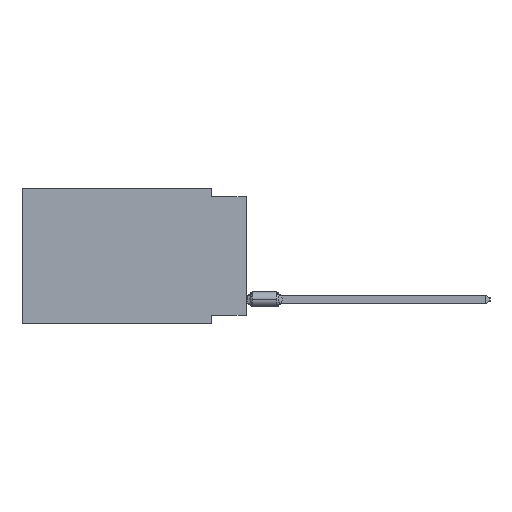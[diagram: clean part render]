
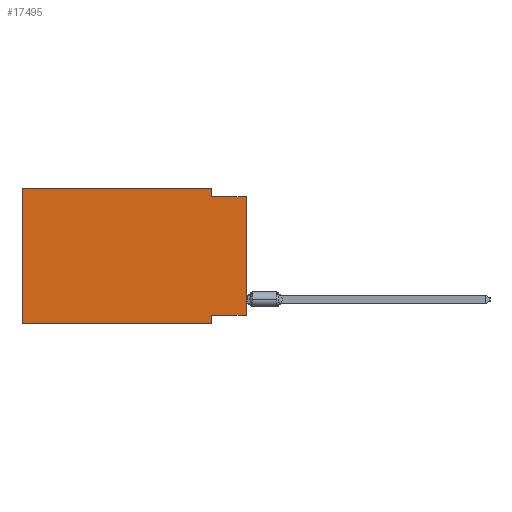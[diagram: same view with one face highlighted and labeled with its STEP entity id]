
A CAD part, left-side view. The second image highlights one B-rep face of the part: STEP entity #17495.
In plain terms, the highlighted planar face has unit normal (-1, 0, 0).
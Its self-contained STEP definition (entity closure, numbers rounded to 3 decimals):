
#126 = VERTEX_POINT ( 'NONE', #58675 ) ;
#635 = VERTEX_POINT ( 'NONE', #7079 ) ;
#2774 = CARTESIAN_POINT ( 'NONE',  ( 0., 0., -9.271 ) ) ;
#3363 = EDGE_CURVE ( 'NONE', #635, #11653, #28227, .T. ) ;
#3423 = LINE ( 'NONE', #3728, #13089 ) ;
#3728 = CARTESIAN_POINT ( 'NONE',  ( 0., 16.383, 0. ) ) ;
#4546 = ORIENTED_EDGE ( 'NONE', *, *, #44623, .F. ) ;
#6617 = AXIS2_PLACEMENT_3D ( 'NONE', #57399, #61791, #23849 ) ;
#7079 = CARTESIAN_POINT ( 'NONE',  ( 0., 2.54, -9.271 ) ) ;
#9538 = DIRECTION ( 'NONE',  ( 0., -1., 0. ) ) ;
#10046 = CARTESIAN_POINT ( 'NONE',  ( 0., 0., 0. ) ) ;
#10373 = DIRECTION ( 'NONE',  ( 0., 0., 1. ) ) ;
#10592 = CARTESIAN_POINT ( 'NONE',  ( 0., 2.54, 0. ) ) ;
#11311 = ORIENTED_EDGE ( 'NONE', *, *, #11532, .F. ) ;
#11532 = EDGE_CURVE ( 'NONE', #30861, #30033, #38598, .T. ) ;
#11653 = VERTEX_POINT ( 'NONE', #49554 ) ;
#12289 = VERTEX_POINT ( 'NONE', #34632 ) ;
#13089 = VECTOR ( 'NONE', #22614, 1000. ) ;
#13993 = LINE ( 'NONE', #18708, #18379 ) ;
#14988 = DIRECTION ( 'NONE',  ( 0., -1., 0. ) ) ;
#15938 = CARTESIAN_POINT ( 'NONE',  ( 0., 0., -0.635 ) ) ;
#17495 = ADVANCED_FACE ( 'NONE', ( #47383 ), #42677, .F. ) ;
#18379 = VECTOR ( 'NONE', #28171, 1000. ) ;
#18708 = CARTESIAN_POINT ( 'NONE',  ( 0., 2.54, 0. ) ) ;
#19190 = ORIENTED_EDGE ( 'NONE', *, *, #34098, .T. ) ;
#19692 = CARTESIAN_POINT ( 'NONE',  ( 0., 16.383, -9.906 ) ) ;
#21379 = CARTESIAN_POINT ( 'NONE',  ( 0., 2.54, -0.635 ) ) ;
#21733 = ORIENTED_EDGE ( 'NONE', *, *, #28636, .F. ) ;
#21975 = DIRECTION ( 'NONE',  ( 0., 1., 0. ) ) ;
#22614 = DIRECTION ( 'NONE',  ( 0., 0., 1. ) ) ;
#23849 = DIRECTION ( 'NONE',  ( 0., 0., -1. ) ) ;
#24661 = LINE ( 'NONE', #43797, #53331 ) ;
#25345 = CARTESIAN_POINT ( 'NONE',  ( 0., 16.383, -9.906 ) ) ;
#28171 = DIRECTION ( 'NONE',  ( 0., 0., -1. ) ) ;
#28227 = LINE ( 'NONE', #42636, #32324 ) ;
#28462 = ORIENTED_EDGE ( 'NONE', *, *, #43310, .F. ) ;
#28636 = EDGE_CURVE ( 'NONE', #126, #49443, #24661, .T. ) ;
#29836 = DIRECTION ( 'NONE',  ( 0., -1., 0. ) ) ;
#29980 = ORIENTED_EDGE ( 'NONE', *, *, #3363, .F. ) ;
#30033 = VERTEX_POINT ( 'NONE', #15938 ) ;
#30861 = VERTEX_POINT ( 'NONE', #21379 ) ;
#31640 = VECTOR ( 'NONE', #14988, 1000. ) ;
#32319 = DIRECTION ( 'NONE',  ( 0., 0., -1. ) ) ;
#32324 = VECTOR ( 'NONE', #32319, 1000. ) ;
#34098 = EDGE_CURVE ( 'NONE', #12289, #30033, #39877, .T. ) ;
#34632 = CARTESIAN_POINT ( 'NONE',  ( 0., 0., -9.271 ) ) ;
#34935 = ORIENTED_EDGE ( 'NONE', *, *, #39458, .F. ) ;
#37427 = VECTOR ( 'NONE', #29836, 1000. ) ;
#38147 = VECTOR ( 'NONE', #21975, 1000. ) ;
#38598 = LINE ( 'NONE', #39234, #37427 ) ;
#39234 = CARTESIAN_POINT ( 'NONE',  ( 0., 0., -0.635 ) ) ;
#39458 = EDGE_CURVE ( 'NONE', #49443, #30861, #13993, .T. ) ;
#39877 = LINE ( 'NONE', #10046, #51987 ) ;
#41455 = ORIENTED_EDGE ( 'NONE', *, *, #48161, .T. ) ;
#42636 = CARTESIAN_POINT ( 'NONE',  ( 0., 2.54, -9.906 ) ) ;
#42677 = PLANE ( 'NONE',  #6617 ) ;
#43310 = EDGE_CURVE ( 'NONE', #12289, #635, #55539, .T. ) ;
#43564 = LINE ( 'NONE', #19692, #31640 ) ;
#43797 = CARTESIAN_POINT ( 'NONE',  ( 0., 16.383, 0. ) ) ;
#44623 = EDGE_CURVE ( 'NONE', #55378, #126, #3423, .T. ) ;
#47383 = FACE_OUTER_BOUND ( 'NONE', #56449, .T. ) ;
#48161 = EDGE_CURVE ( 'NONE', #55378, #11653, #43564, .T. ) ;
#49443 = VERTEX_POINT ( 'NONE', #10592 ) ;
#49554 = CARTESIAN_POINT ( 'NONE',  ( 0., 2.54, -9.906 ) ) ;
#51987 = VECTOR ( 'NONE', #10373, 1000. ) ;
#53331 = VECTOR ( 'NONE', #9538, 1000. ) ;
#55378 = VERTEX_POINT ( 'NONE', #25345 ) ;
#55539 = LINE ( 'NONE', #2774, #38147 ) ;
#56449 = EDGE_LOOP ( 'NONE', ( #19190, #11311, #34935, #21733, #4546, #41455, #29980, #28462 ) ) ;
#57399 = CARTESIAN_POINT ( 'NONE',  ( 0., 16.383, 0. ) ) ;
#58675 = CARTESIAN_POINT ( 'NONE',  ( 0., 16.383, 0. ) ) ;
#61791 = DIRECTION ( 'NONE',  ( 1., 0., 0. ) ) ;
